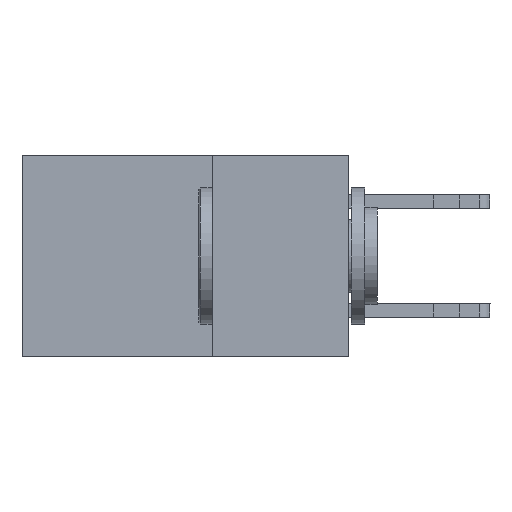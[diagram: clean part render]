
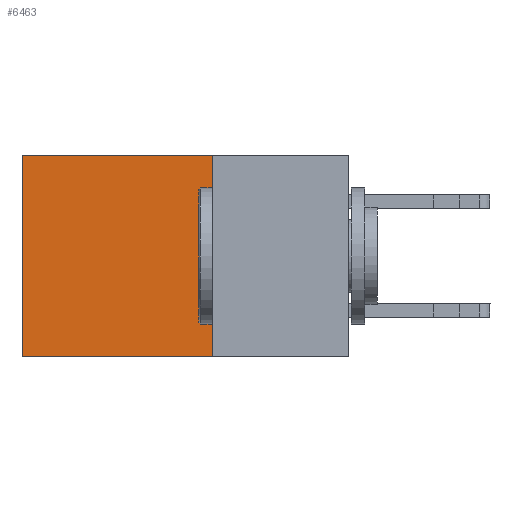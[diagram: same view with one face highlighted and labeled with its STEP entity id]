
A CAD part, left-side view. The second image highlights one B-rep face of the part: STEP entity #6463.
In plain terms, the highlighted planar face has unit normal (-1, 0, 0).
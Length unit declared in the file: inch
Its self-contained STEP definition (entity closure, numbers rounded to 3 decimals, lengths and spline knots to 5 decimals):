
#13 = LINE ( 'NONE', #4147, #2740 ) ;
#31 = ORIENTED_EDGE ( 'NONE', *, *, #12243, .F. ) ;
#141 = VERTEX_POINT ( 'NONE', #2195 ) ;
#167 = EDGE_LOOP ( 'NONE', ( #6296, #31, #2568, #317 ) ) ;
#178 = CARTESIAN_POINT ( 'NONE',  ( 0.2615, 0.25, -0.37 ) ) ;
#317 = ORIENTED_EDGE ( 'NONE', *, *, #7932, .T. ) ;
#1040 = LINE ( 'NONE', #7309, #3416 ) ;
#1648 = VECTOR ( 'NONE', #11672, 39.37008 ) ;
#1829 = CARTESIAN_POINT ( 'NONE',  ( 0.2615, 0.6, 0. ) ) ;
#2195 = CARTESIAN_POINT ( 'NONE',  ( 0.2615, 0.6, -0.37 ) ) ;
#2568 = ORIENTED_EDGE ( 'NONE', *, *, #6556, .F. ) ;
#2740 = VECTOR ( 'NONE', #4192, 39.37008 ) ;
#3416 = VECTOR ( 'NONE', #8311, 39.37008 ) ;
#3756 = VERTEX_POINT ( 'NONE', #1829 ) ;
#3853 = VERTEX_POINT ( 'NONE', #9814 ) ;
#3867 = CARTESIAN_POINT ( 'NONE',  ( 0.2615, 0.25, -0.37 ) ) ;
#4147 = CARTESIAN_POINT ( 'NONE',  ( 0.2615, 0.25, 0. ) ) ;
#4192 = DIRECTION ( 'NONE',  ( 0., 1., 0. ) ) ;
#4414 = CARTESIAN_POINT ( 'NONE',  ( 0.2615, 0.25, 0. ) ) ;
#4664 = LINE ( 'NONE', #3867, #1648 ) ;
#6296 = ORIENTED_EDGE ( 'NONE', *, *, #11903, .T. ) ;
#6463 = ADVANCED_FACE ( 'NONE', ( #7581 ), #12712, .F. ) ;
#6556 = EDGE_CURVE ( 'NONE', #10653, #3853, #9000, .T. ) ;
#7309 = CARTESIAN_POINT ( 'NONE',  ( 0.2615, 0.6, -0.37 ) ) ;
#7581 = FACE_OUTER_BOUND ( 'NONE', #167, .T. ) ;
#7886 = AXIS2_PLACEMENT_3D ( 'NONE', #178, #12685, #12674 ) ;
#7932 = EDGE_CURVE ( 'NONE', #10653, #3756, #13, .T. ) ;
#8311 = DIRECTION ( 'NONE',  ( 0., 0., -1. ) ) ;
#9000 = LINE ( 'NONE', #12284, #11245 ) ;
#9814 = CARTESIAN_POINT ( 'NONE',  ( 0.2615, 0.25, -0.37 ) ) ;
#10653 = VERTEX_POINT ( 'NONE', #4414 ) ;
#11245 = VECTOR ( 'NONE', #12074, 39.37008 ) ;
#11672 = DIRECTION ( 'NONE',  ( 0., 1., 0. ) ) ;
#11903 = EDGE_CURVE ( 'NONE', #3756, #141, #1040, .T. ) ;
#12074 = DIRECTION ( 'NONE',  ( 0., 0., -1. ) ) ;
#12243 = EDGE_CURVE ( 'NONE', #3853, #141, #4664, .T. ) ;
#12284 = CARTESIAN_POINT ( 'NONE',  ( 0.2615, 0.25, -0.37 ) ) ;
#12674 = DIRECTION ( 'NONE',  ( 0., 0., -1. ) ) ;
#12685 = DIRECTION ( 'NONE',  ( 1., 0., 0. ) ) ;
#12712 = PLANE ( 'NONE',  #7886 ) ;
